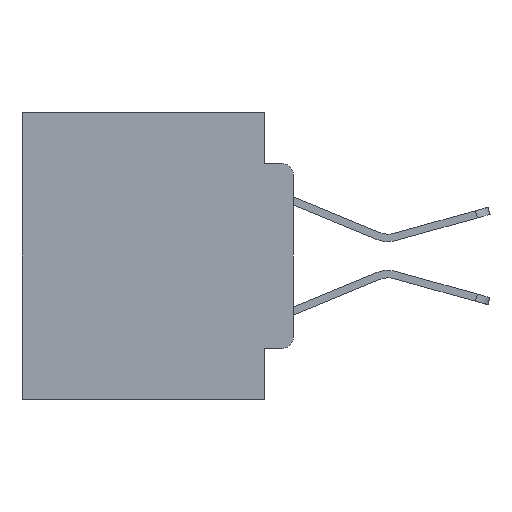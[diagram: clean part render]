
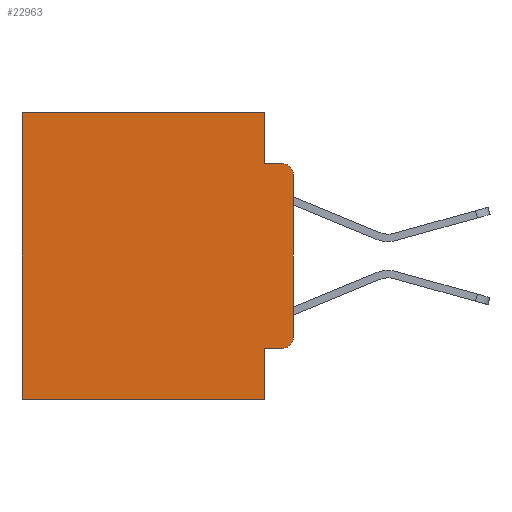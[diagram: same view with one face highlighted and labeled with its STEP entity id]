
A CAD part, left-side view. The second image highlights one B-rep face of the part: STEP entity #22963.
In plain terms, the highlighted planar face has unit normal (-1, 0, 0).
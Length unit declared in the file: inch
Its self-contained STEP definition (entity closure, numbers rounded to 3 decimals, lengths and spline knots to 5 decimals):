
#346 = EDGE_CURVE ( 'NONE', #5216, #25415, #9507, .T. ) ;
#1632 = VECTOR ( 'NONE', #24771, 39.37008 ) ;
#1875 = EDGE_CURVE ( 'NONE', #5473, #7430, #23594, .T. ) ;
#1960 = VERTEX_POINT ( 'NONE', #15093 ) ;
#2121 = DIRECTION ( 'NONE',  ( -1., 0., 0. ) ) ;
#2159 = VECTOR ( 'NONE', #9760, 39.37008 ) ;
#2162 = DIRECTION ( 'NONE',  ( 0., -1., 0. ) ) ;
#2366 = ORIENTED_EDGE ( 'NONE', *, *, #346, .F. ) ;
#2493 = AXIS2_PLACEMENT_3D ( 'NONE', #18391, #5691, #20503 ) ;
#3039 = ORIENTED_EDGE ( 'NONE', *, *, #9139, .T. ) ;
#3067 = ORIENTED_EDGE ( 'NONE', *, *, #26213, .T. ) ;
#3357 = VERTEX_POINT ( 'NONE', #6710 ) ;
#3376 = EDGE_CURVE ( 'NONE', #25729, #5216, #21558, .T. ) ;
#3457 = VECTOR ( 'NONE', #12224, 39.37008 ) ;
#3509 = PLANE ( 'NONE',  #2493 ) ;
#3817 = VECTOR ( 'NONE', #2162, 39.37008 ) ;
#3938 = EDGE_CURVE ( 'NONE', #8250, #7430, #14601, .T. ) ;
#3975 = CARTESIAN_POINT ( 'NONE',  ( 0.298, 0.473, 0. ) ) ;
#4019 = DIRECTION ( 'NONE',  ( 0., 1., 0. ) ) ;
#5216 = VERTEX_POINT ( 'NONE', #6798 ) ;
#5371 = EDGE_CURVE ( 'NONE', #23359, #8250, #25419, .T. ) ;
#5473 = VERTEX_POINT ( 'NONE', #22980 ) ;
#5691 = DIRECTION ( 'NONE',  ( 1., 0., 0. ) ) ;
#5750 = VECTOR ( 'NONE', #6731, 39.37008 ) ;
#6710 = CARTESIAN_POINT ( 'NONE',  ( 0.298, 0.051, -0.5 ) ) ;
#6731 = DIRECTION ( 'NONE',  ( 0., 0., -1. ) ) ;
#6798 = CARTESIAN_POINT ( 'NONE',  ( 0.298, 0.051, -0.0885 ) ) ;
#7430 = VERTEX_POINT ( 'NONE', #15754 ) ;
#7435 = CARTESIAN_POINT ( 'NONE',  ( 0.298, 0.473, -0.5 ) ) ;
#8202 = EDGE_CURVE ( 'NONE', #25729, #1960, #21126, .T. ) ;
#8250 = VERTEX_POINT ( 'NONE', #22668 ) ;
#8427 = LINE ( 'NONE', #20985, #19676 ) ;
#8808 = ORIENTED_EDGE ( 'NONE', *, *, #1875, .F. ) ;
#9139 = EDGE_CURVE ( 'NONE', #1960, #23499, #9851, .T. ) ;
#9443 = ORIENTED_EDGE ( 'NONE', *, *, #8202, .T. ) ;
#9507 = LINE ( 'NONE', #10767, #3817 ) ;
#9760 = DIRECTION ( 'NONE',  ( 0., -1., 0. ) ) ;
#9851 = LINE ( 'NONE', #3975, #3457 ) ;
#10353 = VECTOR ( 'NONE', #18598, 39.37008 ) ;
#10449 = CARTESIAN_POINT ( 'NONE',  ( 0.298, 0.051, -0.4115 ) ) ;
#10578 = EDGE_CURVE ( 'NONE', #23359, #3357, #12076, .T. ) ;
#10767 = CARTESIAN_POINT ( 'NONE',  ( 0.298, 0.051, -0.0885 ) ) ;
#11419 = CARTESIAN_POINT ( 'NONE',  ( 0.298, 0., 0. ) ) ;
#11756 = ORIENTED_EDGE ( 'NONE', *, *, #3938, .T. ) ;
#11883 = AXIS2_PLACEMENT_3D ( 'NONE', #11923, #15117, #14514 ) ;
#11923 = CARTESIAN_POINT ( 'NONE',  ( 0.298, 0.02, -0.3915 ) ) ;
#12076 = LINE ( 'NONE', #25619, #5750 ) ;
#12224 = DIRECTION ( 'NONE',  ( 0., 0., -1. ) ) ;
#12394 = CIRCLE ( 'NONE', #18645, 0.02 ) ;
#12472 = FACE_OUTER_BOUND ( 'NONE', #13028, .T. ) ;
#13028 = EDGE_LOOP ( 'NONE', ( #8808, #3067, #2366, #24284, #9443, #3039, #23604, #18035, #17373, #11756 ) ) ;
#14514 = DIRECTION ( 'NONE',  ( 0., 0., -1. ) ) ;
#14601 = CIRCLE ( 'NONE', #11883, 0.02 ) ;
#14951 = CARTESIAN_POINT ( 'NONE',  ( 0.298, 0.02, -0.1085 ) ) ;
#15093 = CARTESIAN_POINT ( 'NONE',  ( 0.298, 0.473, 0. ) ) ;
#15117 = DIRECTION ( 'NONE',  ( -1., 0., 0. ) ) ;
#15483 = VECTOR ( 'NONE', #16345, 39.37008 ) ;
#15754 = CARTESIAN_POINT ( 'NONE',  ( 0.298, 0., -0.3915 ) ) ;
#16345 = DIRECTION ( 'NONE',  ( 0., 1., 0. ) ) ;
#17087 = DIRECTION ( 'NONE',  ( 0., 0., -1. ) ) ;
#17373 = ORIENTED_EDGE ( 'NONE', *, *, #5371, .T. ) ;
#17526 = CARTESIAN_POINT ( 'NONE',  ( 0.298, 0.051, -0.4115 ) ) ;
#18035 = ORIENTED_EDGE ( 'NONE', *, *, #10578, .F. ) ;
#18259 = CARTESIAN_POINT ( 'NONE',  ( 0.298, 0.051, 0. ) ) ;
#18391 = CARTESIAN_POINT ( 'NONE',  ( 0.298, 0., 0. ) ) ;
#18598 = DIRECTION ( 'NONE',  ( 0., 0., -1. ) ) ;
#18645 = AXIS2_PLACEMENT_3D ( 'NONE', #14951, #2121, #17087 ) ;
#19676 = VECTOR ( 'NONE', #4019, 39.37008 ) ;
#20503 = DIRECTION ( 'NONE',  ( 0., 0., -1. ) ) ;
#20714 = CARTESIAN_POINT ( 'NONE',  ( 0.298, 0.02, -0.0885 ) ) ;
#20985 = CARTESIAN_POINT ( 'NONE',  ( 0.298, 0., -0.5 ) ) ;
#21126 = LINE ( 'NONE', #11419, #15483 ) ;
#21558 = LINE ( 'NONE', #18259, #10353 ) ;
#21702 = CARTESIAN_POINT ( 'NONE',  ( 0.298, 0.051, 0. ) ) ;
#22668 = CARTESIAN_POINT ( 'NONE',  ( 0.298, 0.02, -0.4115 ) ) ;
#22963 = ADVANCED_FACE ( 'NONE', ( #12472 ), #3509, .F. ) ;
#22980 = CARTESIAN_POINT ( 'NONE',  ( 0.298, 0., -0.1085 ) ) ;
#23359 = VERTEX_POINT ( 'NONE', #17526 ) ;
#23499 = VERTEX_POINT ( 'NONE', #7435 ) ;
#23594 = LINE ( 'NONE', #24737, #1632 ) ;
#23604 = ORIENTED_EDGE ( 'NONE', *, *, #25505, .F. ) ;
#24284 = ORIENTED_EDGE ( 'NONE', *, *, #3376, .F. ) ;
#24737 = CARTESIAN_POINT ( 'NONE',  ( 0.298, 0., 0. ) ) ;
#24771 = DIRECTION ( 'NONE',  ( 0., 0., -1. ) ) ;
#25415 = VERTEX_POINT ( 'NONE', #20714 ) ;
#25419 = LINE ( 'NONE', #10449, #2159 ) ;
#25505 = EDGE_CURVE ( 'NONE', #3357, #23499, #8427, .T. ) ;
#25619 = CARTESIAN_POINT ( 'NONE',  ( 0.298, 0.051, 0. ) ) ;
#25729 = VERTEX_POINT ( 'NONE', #21702 ) ;
#26213 = EDGE_CURVE ( 'NONE', #5473, #25415, #12394, .T. ) ;
